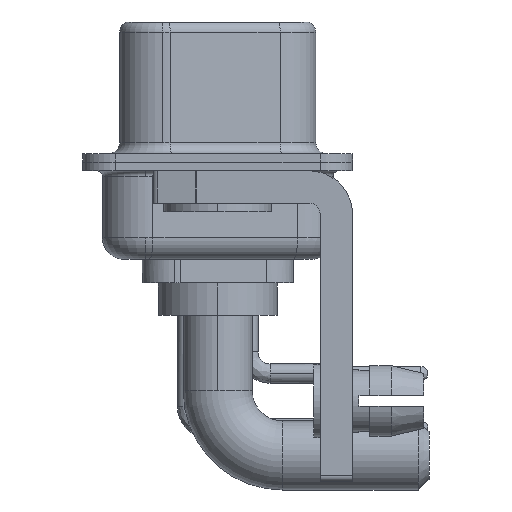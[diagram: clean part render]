
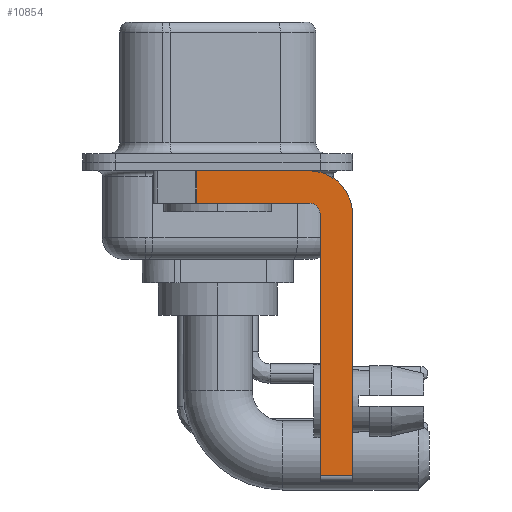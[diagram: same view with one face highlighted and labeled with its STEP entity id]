
A CAD part, left-side view. The second image highlights one B-rep face of the part: STEP entity #10854.
In plain terms, the highlighted planar face has unit normal (-1, 0, 0).
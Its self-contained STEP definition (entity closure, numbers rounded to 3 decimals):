
#124 = LINE ( 'NONE', #3784, #7542 ) ;
#247 = VECTOR ( 'NONE', #15009, 1000. ) ;
#327 = VERTEX_POINT ( 'NONE', #13177 ) ;
#1421 = EDGE_CURVE ( 'NONE', #12486, #9517, #23259, .T. ) ;
#1452 = DIRECTION ( 'NONE',  ( 0., 0., 1. ) ) ;
#1836 = DIRECTION ( 'NONE',  ( 0., 1., 0. ) ) ;
#1838 = DIRECTION ( 'NONE',  ( 0., 0., -1. ) ) ;
#2825 = EDGE_CURVE ( 'NONE', #16607, #327, #10900, .T. ) ;
#2955 = ORIENTED_EDGE ( 'NONE', *, *, #8460, .T. ) ;
#3784 = CARTESIAN_POINT ( 'NONE',  ( -2.9, -4.25, -14.55 ) ) ;
#3932 = ORIENTED_EDGE ( 'NONE', *, *, #2825, .T. ) ;
#4044 = EDGE_CURVE ( 'NONE', #12367, #12822, #21384, .T. ) ;
#4360 = PLANE ( 'NONE',  #11095 ) ;
#4494 = DIRECTION ( 'NONE',  ( 1., 0., 0. ) ) ;
#4838 = ORIENTED_EDGE ( 'NONE', *, *, #8672, .F. ) ;
#5302 = EDGE_LOOP ( 'NONE', ( #5812, #3932, #4838, #7953, #19183, #2955, #12132, #20532 ) ) ;
#5812 = ORIENTED_EDGE ( 'NONE', *, *, #21523, .F. ) ;
#5813 = DIRECTION ( 'NONE',  ( 0., 0., -1. ) ) ;
#7542 = VECTOR ( 'NONE', #15743, 1000. ) ;
#7953 = ORIENTED_EDGE ( 'NONE', *, *, #8485, .F. ) ;
#8015 = CARTESIAN_POINT ( 'NONE',  ( -2.9, -4.75, -2.4 ) ) ;
#8186 = CARTESIAN_POINT ( 'NONE',  ( -2.9, -6.25, -2.4 ) ) ;
#8460 = EDGE_CURVE ( 'NONE', #12486, #11052, #124, .T. ) ;
#8485 = EDGE_CURVE ( 'NONE', #9517, #10859, #21481, .T. ) ;
#8672 = EDGE_CURVE ( 'NONE', #10859, #327, #10769, .T. ) ;
#8909 = CARTESIAN_POINT ( 'NONE',  ( -2.9, 3., -0.4 ) ) ;
#9517 = VERTEX_POINT ( 'NONE', #8015 ) ;
#9596 = LINE ( 'NONE', #8186, #247 ) ;
#10322 = DIRECTION ( 'NONE',  ( -1., 0., 0. ) ) ;
#10769 = LINE ( 'NONE', #17957, #22628 ) ;
#10784 = LINE ( 'NONE', #8909, #13424 ) ;
#10854 = ADVANCED_FACE ( 'NONE', ( #13658 ), #4360, .F. ) ;
#10859 = VERTEX_POINT ( 'NONE', #17086 ) ;
#10900 = LINE ( 'NONE', #16427, #19534 ) ;
#11052 = VERTEX_POINT ( 'NONE', #21116 ) ;
#11095 = AXIS2_PLACEMENT_3D ( 'NONE', #16854, #4494, #11892 ) ;
#11349 = CARTESIAN_POINT ( 'NONE',  ( -2.9, -4.25, -2.4 ) ) ;
#11892 = DIRECTION ( 'NONE',  ( 0., 0., -1. ) ) ;
#12043 = CARTESIAN_POINT ( 'NONE',  ( -2.9, -6.25, -2.4 ) ) ;
#12132 = ORIENTED_EDGE ( 'NONE', *, *, #20562, .F. ) ;
#12367 = VERTEX_POINT ( 'NONE', #19821 ) ;
#12486 = VERTEX_POINT ( 'NONE', #18504 ) ;
#12540 = DIRECTION ( 'NONE',  ( 0., -1., 0. ) ) ;
#12822 = VERTEX_POINT ( 'NONE', #12043 ) ;
#13177 = CARTESIAN_POINT ( 'NONE',  ( -2.9, 0.978, -1.9 ) ) ;
#13424 = VECTOR ( 'NONE', #12540, 1000. ) ;
#13658 = FACE_OUTER_BOUND ( 'NONE', #5302, .T. ) ;
#15009 = DIRECTION ( 'NONE',  ( 0., 0., -1. ) ) ;
#15062 = AXIS2_PLACEMENT_3D ( 'NONE', #21059, #10322, #15508 ) ;
#15508 = DIRECTION ( 'NONE',  ( 0., 0., 1. ) ) ;
#15743 = DIRECTION ( 'NONE',  ( 0., -1., 0. ) ) ;
#16427 = CARTESIAN_POINT ( 'NONE',  ( -2.9, 0.978, -1.9 ) ) ;
#16607 = VERTEX_POINT ( 'NONE', #19298 ) ;
#16854 = CARTESIAN_POINT ( 'NONE',  ( -2.9, -4.25, -2.4 ) ) ;
#17086 = CARTESIAN_POINT ( 'NONE',  ( -2.9, -4.25, -1.9 ) ) ;
#17575 = CARTESIAN_POINT ( 'NONE',  ( -2.9, -4.75, -14.8 ) ) ;
#17957 = CARTESIAN_POINT ( 'NONE',  ( -2.9, -4.25, -1.9 ) ) ;
#18504 = CARTESIAN_POINT ( 'NONE',  ( -2.9, -4.75, -14.55 ) ) ;
#18735 = AXIS2_PLACEMENT_3D ( 'NONE', #11349, #22100, #5813 ) ;
#19183 = ORIENTED_EDGE ( 'NONE', *, *, #1421, .F. ) ;
#19298 = CARTESIAN_POINT ( 'NONE',  ( -2.9, 0.978, -0.4 ) ) ;
#19534 = VECTOR ( 'NONE', #1838, 1000. ) ;
#19821 = CARTESIAN_POINT ( 'NONE',  ( -2.9, -4.25, -0.4 ) ) ;
#20532 = ORIENTED_EDGE ( 'NONE', *, *, #4044, .F. ) ;
#20562 = EDGE_CURVE ( 'NONE', #12822, #11052, #9596, .T. ) ;
#21059 = CARTESIAN_POINT ( 'NONE',  ( -2.9, -4.25, -2.4 ) ) ;
#21116 = CARTESIAN_POINT ( 'NONE',  ( -2.9, -6.25, -14.55 ) ) ;
#21208 = VECTOR ( 'NONE', #1452, 1000. ) ;
#21384 = CIRCLE ( 'NONE', #18735, 2. ) ;
#21481 = CIRCLE ( 'NONE', #15062, 0.5 ) ;
#21523 = EDGE_CURVE ( 'NONE', #16607, #12367, #10784, .T. ) ;
#22100 = DIRECTION ( 'NONE',  ( 1., 0., 0. ) ) ;
#22628 = VECTOR ( 'NONE', #1836, 1000. ) ;
#23259 = LINE ( 'NONE', #17575, #21208 ) ;
